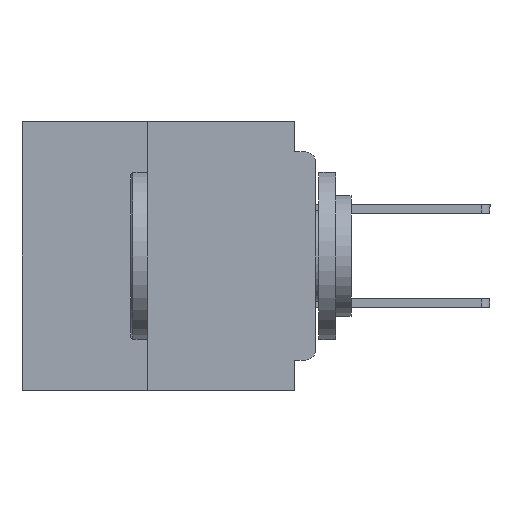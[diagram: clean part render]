
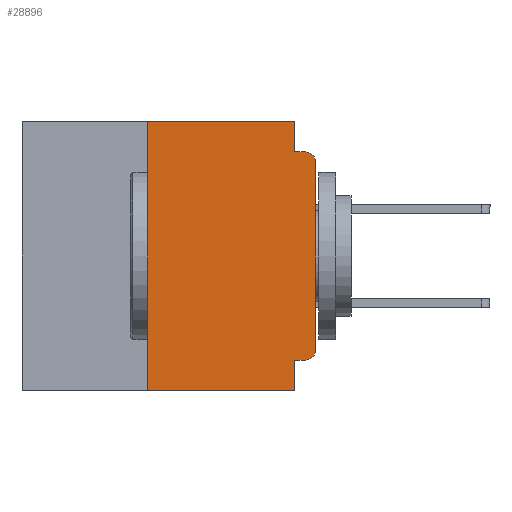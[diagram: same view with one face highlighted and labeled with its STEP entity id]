
A CAD part, left-side view. The second image highlights one B-rep face of the part: STEP entity #28896.
In plain terms, the highlighted planar face has unit normal (-1, 0, 0).
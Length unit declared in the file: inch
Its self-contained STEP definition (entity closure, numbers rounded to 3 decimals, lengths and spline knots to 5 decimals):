
#274 = ORIENTED_EDGE ( 'NONE', *, *, #49282, .F. ) ;
#431 = VERTEX_POINT ( 'NONE', #52419 ) ;
#772 = ORIENTED_EDGE ( 'NONE', *, *, #46919, .T. ) ;
#837 = ORIENTED_EDGE ( 'NONE', *, *, #16861, .F. ) ;
#1027 = LINE ( 'NONE', #21792, #25843 ) ;
#1029 = ORIENTED_EDGE ( 'NONE', *, *, #35502, .F. ) ;
#1255 = AXIS2_PLACEMENT_3D ( 'NONE', #36737, #10626, #41067 ) ;
#1888 = VECTOR ( 'NONE', #8723, 39.37008 ) ;
#2190 = CARTESIAN_POINT ( 'NONE',  ( 0., 0., -0.355 ) ) ;
#2281 = VERTEX_POINT ( 'NONE', #24789 ) ;
#2370 = VECTOR ( 'NONE', #6774, 39.37008 ) ;
#3648 = VERTEX_POINT ( 'NONE', #6330 ) ;
#4426 = VECTOR ( 'NONE', #55496, 39.37008 ) ;
#4738 = DIRECTION ( 'NONE',  ( 1., 0., 0. ) ) ;
#5303 = CARTESIAN_POINT ( 'NONE',  ( 0., 0.25, -0.4 ) ) ;
#5662 = VERTEX_POINT ( 'NONE', #52578 ) ;
#5802 = LINE ( 'NONE', #5303, #50611 ) ;
#5835 = CARTESIAN_POINT ( 'NONE',  ( 0., 0.031, -0.355 ) ) ;
#6330 = CARTESIAN_POINT ( 'NONE',  ( 0., 0.25, -0.4 ) ) ;
#6774 = DIRECTION ( 'NONE',  ( 0., 1., 0. ) ) ;
#8723 = DIRECTION ( 'NONE',  ( 0., -1., 0. ) ) ;
#9267 = VERTEX_POINT ( 'NONE', #11305 ) ;
#9965 = FACE_OUTER_BOUND ( 'NONE', #52415, .T. ) ;
#10626 = DIRECTION ( 'NONE',  ( -1., 0., 0. ) ) ;
#11305 = CARTESIAN_POINT ( 'NONE',  ( 0., 0., -0.34 ) ) ;
#12662 = CARTESIAN_POINT ( 'NONE',  ( 0., 0., 0. ) ) ;
#13084 = VERTEX_POINT ( 'NONE', #49153 ) ;
#13146 = VERTEX_POINT ( 'NONE', #45217 ) ;
#13749 = EDGE_CURVE ( 'NONE', #48740, #9267, #45638, .T. ) ;
#14101 = LINE ( 'NONE', #2190, #2370 ) ;
#14781 = ORIENTED_EDGE ( 'NONE', *, *, #13749, .T. ) ;
#15510 = ORIENTED_EDGE ( 'NONE', *, *, #37606, .T. ) ;
#16596 = CARTESIAN_POINT ( 'NONE',  ( 0., 0.031, -0.4 ) ) ;
#16861 = EDGE_CURVE ( 'NONE', #431, #2281, #37947, .T. ) ;
#17624 = AXIS2_PLACEMENT_3D ( 'NONE', #44530, #18655, #48832 ) ;
#17686 = PLANE ( 'NONE',  #21001 ) ;
#18655 = DIRECTION ( 'NONE',  ( -1., 0., 0. ) ) ;
#19761 = VECTOR ( 'NONE', #55663, 39.37008 ) ;
#20074 = VECTOR ( 'NONE', #46111, 39.37008 ) ;
#20717 = ORIENTED_EDGE ( 'NONE', *, *, #39157, .F. ) ;
#21001 = AXIS2_PLACEMENT_3D ( 'NONE', #48070, #4738, #35346 ) ;
#21454 = LINE ( 'NONE', #41830, #20074 ) ;
#21792 = CARTESIAN_POINT ( 'NONE',  ( 0., 0.031, 0. ) ) ;
#24081 = VECTOR ( 'NONE', #34076, 39.37008 ) ;
#24789 = CARTESIAN_POINT ( 'NONE',  ( 0., 0.015, -0.045 ) ) ;
#24793 = CARTESIAN_POINT ( 'NONE',  ( 0., 0.031, 0. ) ) ;
#25843 = VECTOR ( 'NONE', #51878, 39.37008 ) ;
#28382 = EDGE_CURVE ( 'NONE', #41972, #431, #1027, .T. ) ;
#28836 = ORIENTED_EDGE ( 'NONE', *, *, #48110, .T. ) ;
#28896 = ADVANCED_FACE ( 'NONE', ( #9965 ), #17686, .F. ) ;
#29611 = VERTEX_POINT ( 'NONE', #5835 ) ;
#34076 = DIRECTION ( 'NONE',  ( 0., 0., -1. ) ) ;
#34210 = CARTESIAN_POINT ( 'NONE',  ( 0., 0., -0.045 ) ) ;
#35346 = DIRECTION ( 'NONE',  ( 0., 0., -1. ) ) ;
#35502 = EDGE_CURVE ( 'NONE', #13146, #41972, #21454, .T. ) ;
#35603 = LINE ( 'NONE', #16596, #24081 ) ;
#36737 = CARTESIAN_POINT ( 'NONE',  ( 0., 0.015, -0.34 ) ) ;
#37606 = EDGE_CURVE ( 'NONE', #13084, #2281, #47824, .T. ) ;
#37947 = LINE ( 'NONE', #34210, #4426 ) ;
#38833 = CARTESIAN_POINT ( 'NONE',  ( 0., 0.015, -0.355 ) ) ;
#39157 = EDGE_CURVE ( 'NONE', #29611, #5662, #35603, .T. ) ;
#39592 = ORIENTED_EDGE ( 'NONE', *, *, #28382, .F. ) ;
#40252 = DIRECTION ( 'NONE',  ( 0., 0., 1. ) ) ;
#41067 = DIRECTION ( 'NONE',  ( 0., 0., -1. ) ) ;
#41582 = ORIENTED_EDGE ( 'NONE', *, *, #43026, .F. ) ;
#41830 = CARTESIAN_POINT ( 'NONE',  ( 0., 0.437, 0. ) ) ;
#41972 = VERTEX_POINT ( 'NONE', #24793 ) ;
#42718 = LINE ( 'NONE', #12662, #19761 ) ;
#43026 = EDGE_CURVE ( 'NONE', #48740, #29611, #14101, .T. ) ;
#43485 = CARTESIAN_POINT ( 'NONE',  ( 0., 0.437, -0.4 ) ) ;
#44530 = CARTESIAN_POINT ( 'NONE',  ( 0., 0.015, -0.06 ) ) ;
#45217 = CARTESIAN_POINT ( 'NONE',  ( 0., 0.25, 0. ) ) ;
#45638 = CIRCLE ( 'NONE', #1255, 0.015 ) ;
#46111 = DIRECTION ( 'NONE',  ( 0., -1., 0. ) ) ;
#46794 = LINE ( 'NONE', #43485, #1888 ) ;
#46919 = EDGE_CURVE ( 'NONE', #3648, #5662, #46794, .T. ) ;
#47824 = CIRCLE ( 'NONE', #17624, 0.015 ) ;
#48070 = CARTESIAN_POINT ( 'NONE',  ( 0., 0.437, 0. ) ) ;
#48110 = EDGE_CURVE ( 'NONE', #9267, #13084, #42718, .T. ) ;
#48740 = VERTEX_POINT ( 'NONE', #38833 ) ;
#48832 = DIRECTION ( 'NONE',  ( 0., 0., -1. ) ) ;
#49153 = CARTESIAN_POINT ( 'NONE',  ( 0., 0., -0.06 ) ) ;
#49282 = EDGE_CURVE ( 'NONE', #3648, #13146, #5802, .T. ) ;
#50611 = VECTOR ( 'NONE', #40252, 39.37008 ) ;
#51878 = DIRECTION ( 'NONE',  ( 0., 0., -1. ) ) ;
#52415 = EDGE_LOOP ( 'NONE', ( #28836, #15510, #837, #39592, #1029, #274, #772, #20717, #41582, #14781 ) ) ;
#52419 = CARTESIAN_POINT ( 'NONE',  ( 0., 0.031, -0.045 ) ) ;
#52578 = CARTESIAN_POINT ( 'NONE',  ( 0., 0.031, -0.4 ) ) ;
#55496 = DIRECTION ( 'NONE',  ( 0., -1., 0. ) ) ;
#55663 = DIRECTION ( 'NONE',  ( 0., 0., 1. ) ) ;
